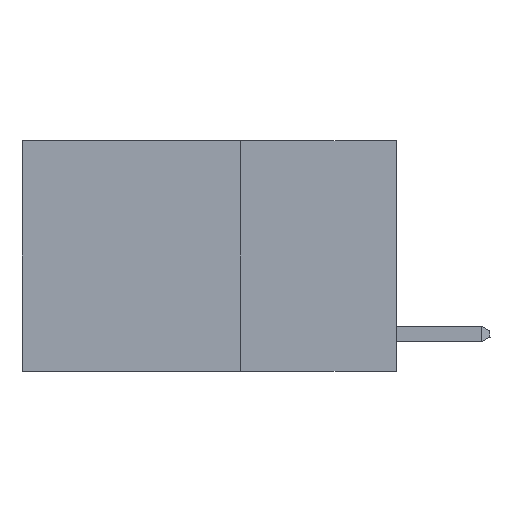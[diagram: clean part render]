
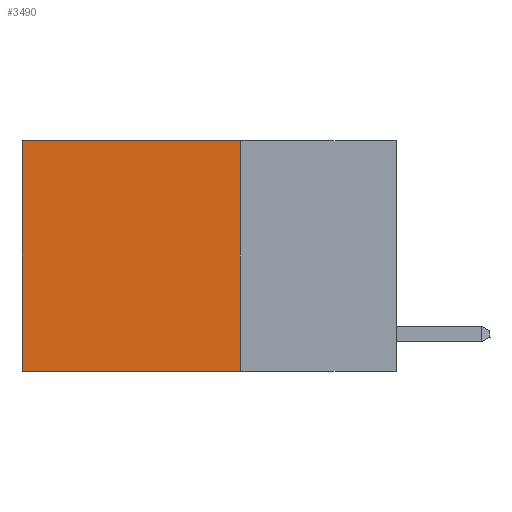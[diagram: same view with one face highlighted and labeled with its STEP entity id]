
A CAD part, left-side view. The second image highlights one B-rep face of the part: STEP entity #3490.
In plain terms, the highlighted planar face has unit normal (-1, 0, 0).
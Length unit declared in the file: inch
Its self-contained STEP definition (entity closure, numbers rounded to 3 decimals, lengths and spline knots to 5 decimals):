
#813 = DIRECTION ( 'NONE',  ( 0., 1., 0. ) ) ;
#1771 = DIRECTION ( 'NONE',  ( 0., 0., -1. ) ) ;
#2989 = DIRECTION ( 'NONE',  ( 1., 0., 0. ) ) ;
#3490 = ADVANCED_FACE ( 'NONE', ( #12950 ), #4983, .F. ) ;
#4983 = PLANE ( 'NONE',  #19843 ) ;
#5166 = EDGE_LOOP ( 'NONE', ( #16563, #7784, #10083, #7830 ) ) ;
#6245 = VERTEX_POINT ( 'NONE', #14399 ) ;
#7038 = EDGE_CURVE ( 'NONE', #16422, #22846, #16970, .T. ) ;
#7396 = VECTOR ( 'NONE', #13713, 39.37008 ) ;
#7784 = ORIENTED_EDGE ( 'NONE', *, *, #26429, .F. ) ;
#7830 = ORIENTED_EDGE ( 'NONE', *, *, #7038, .T. ) ;
#8755 = CARTESIAN_POINT ( 'NONE',  ( 0.2625, 0.6, 0. ) ) ;
#9063 = CARTESIAN_POINT ( 'NONE',  ( 0.2625, 0.25, -0.37 ) ) ;
#9137 = DIRECTION ( 'NONE',  ( 0., 1., 0. ) ) ;
#10083 = ORIENTED_EDGE ( 'NONE', *, *, #24369, .F. ) ;
#10306 = CARTESIAN_POINT ( 'NONE',  ( 0.2625, 0.25, 0. ) ) ;
#10317 = CARTESIAN_POINT ( 'NONE',  ( 0.2625, 0.6, -0.37 ) ) ;
#11167 = LINE ( 'NONE', #9063, #15996 ) ;
#11211 = CARTESIAN_POINT ( 'NONE',  ( 0.2625, 0.25, 0. ) ) ;
#12088 = CARTESIAN_POINT ( 'NONE',  ( 0.2625, 0.6, 0. ) ) ;
#12877 = LINE ( 'NONE', #15798, #7396 ) ;
#12950 = FACE_OUTER_BOUND ( 'NONE', #5166, .T. ) ;
#13713 = DIRECTION ( 'NONE',  ( 0., 0., -1. ) ) ;
#14399 = CARTESIAN_POINT ( 'NONE',  ( 0.2625, 0.25, -0.37 ) ) ;
#14439 = VECTOR ( 'NONE', #1771, 39.37008 ) ;
#14440 = VERTEX_POINT ( 'NONE', #10317 ) ;
#15103 = LINE ( 'NONE', #12088, #14439 ) ;
#15798 = CARTESIAN_POINT ( 'NONE',  ( 0.2625, 0.25, 0. ) ) ;
#15996 = VECTOR ( 'NONE', #813, 39.37008 ) ;
#16422 = VERTEX_POINT ( 'NONE', #10306 ) ;
#16563 = ORIENTED_EDGE ( 'NONE', *, *, #25398, .T. ) ;
#16970 = LINE ( 'NONE', #19421, #21784 ) ;
#17423 = DIRECTION ( 'NONE',  ( 0., 0., -1. ) ) ;
#19421 = CARTESIAN_POINT ( 'NONE',  ( 0.2625, 0.25, 0. ) ) ;
#19843 = AXIS2_PLACEMENT_3D ( 'NONE', #11211, #2989, #17423 ) ;
#21784 = VECTOR ( 'NONE', #9137, 39.37008 ) ;
#22846 = VERTEX_POINT ( 'NONE', #8755 ) ;
#24369 = EDGE_CURVE ( 'NONE', #16422, #6245, #12877, .T. ) ;
#25398 = EDGE_CURVE ( 'NONE', #22846, #14440, #15103, .T. ) ;
#26429 = EDGE_CURVE ( 'NONE', #6245, #14440, #11167, .T. ) ;
